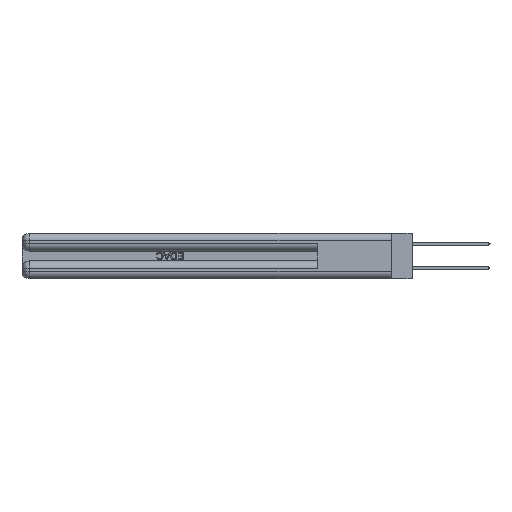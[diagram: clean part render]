
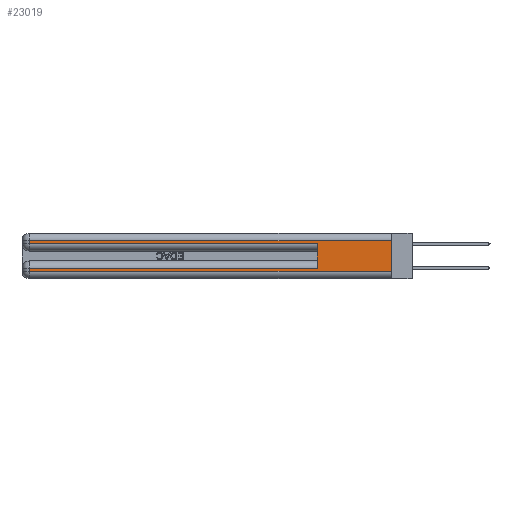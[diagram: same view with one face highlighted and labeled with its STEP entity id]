
A CAD part, left-side view. The second image highlights one B-rep face of the part: STEP entity #23019.
In plain terms, the highlighted planar face has unit normal (-1, 0, 0).
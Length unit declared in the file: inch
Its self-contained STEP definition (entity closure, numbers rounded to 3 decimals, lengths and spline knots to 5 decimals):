
#2296 = VERTEX_POINT ( 'NONE', #18502 ) ;
#3712 = VECTOR ( 'NONE', #10971, 39.37008 ) ;
#4779 = DIRECTION ( 'NONE',  ( 0., 0., -1. ) ) ;
#4962 = LINE ( 'NONE', #7095, #3712 ) ;
#5182 = CARTESIAN_POINT ( 'NONE',  ( 0., 2.94, 0.37 ) ) ;
#5480 = EDGE_CURVE ( 'NONE', #11653, #17614, #48073, .T. ) ;
#6185 = ORIENTED_EDGE ( 'NONE', *, *, #13485, .F. ) ;
#7095 = CARTESIAN_POINT ( 'NONE',  ( 0., 0., 0.06 ) ) ;
#7738 = CARTESIAN_POINT ( 'NONE',  ( 0., 0.6, 0.285 ) ) ;
#10971 = DIRECTION ( 'NONE',  ( 0., -1., 0. ) ) ;
#11653 = VERTEX_POINT ( 'NONE', #35361 ) ;
#11912 = DIRECTION ( 'NONE',  ( 0., 1., 0. ) ) ;
#13485 = EDGE_CURVE ( 'NONE', #11653, #46406, #41781, .T. ) ;
#13730 = EDGE_CURVE ( 'NONE', #17614, #25439, #42348, .T. ) ;
#14300 = CARTESIAN_POINT ( 'NONE',  ( 0., 0., 0.37 ) ) ;
#14472 = ORIENTED_EDGE ( 'NONE', *, *, #40665, .T. ) ;
#14673 = EDGE_CURVE ( 'NONE', #25762, #19172, #30805, .T. ) ;
#16099 = LINE ( 'NONE', #44958, #44363 ) ;
#17614 = VERTEX_POINT ( 'NONE', #29592 ) ;
#18148 = DIRECTION ( 'NONE',  ( 0., 0., -1. ) ) ;
#18502 = CARTESIAN_POINT ( 'NONE',  ( 0., 2.94, 0.06 ) ) ;
#18577 = CARTESIAN_POINT ( 'NONE',  ( 0., 2.94, 0.37 ) ) ;
#19172 = VERTEX_POINT ( 'NONE', #7738 ) ;
#19810 = EDGE_CURVE ( 'NONE', #2296, #46406, #4962, .T. ) ;
#20044 = LINE ( 'NONE', #18577, #49544 ) ;
#20166 = LINE ( 'NONE', #48658, #39418 ) ;
#20925 = ORIENTED_EDGE ( 'NONE', *, *, #19810, .T. ) ;
#21253 = DIRECTION ( 'NONE',  ( 0., 0., 1. ) ) ;
#22101 = ORIENTED_EDGE ( 'NONE', *, *, #5480, .T. ) ;
#22471 = DIRECTION ( 'NONE',  ( 0., 0., -1. ) ) ;
#23019 = ADVANCED_FACE ( 'NONE', ( #25878 ), #37299, .F. ) ;
#23479 = EDGE_LOOP ( 'NONE', ( #6185, #22101, #35210, #14472, #24970, #36206, #28091, #20925 ) ) ;
#24023 = VERTEX_POINT ( 'NONE', #25479 ) ;
#24338 = VECTOR ( 'NONE', #4779, 39.37008 ) ;
#24970 = ORIENTED_EDGE ( 'NONE', *, *, #14673, .F. ) ;
#25439 = VERTEX_POINT ( 'NONE', #44854 ) ;
#25479 = CARTESIAN_POINT ( 'NONE',  ( 0., 2.94, 0.085 ) ) ;
#25762 = VERTEX_POINT ( 'NONE', #31152 ) ;
#25878 = FACE_OUTER_BOUND ( 'NONE', #23479, .T. ) ;
#26979 = DIRECTION ( 'NONE',  ( 0., 0., -1. ) ) ;
#27255 = AXIS2_PLACEMENT_3D ( 'NONE', #14300, #41197, #18148 ) ;
#28091 = ORIENTED_EDGE ( 'NONE', *, *, #32267, .T. ) ;
#29592 = CARTESIAN_POINT ( 'NONE',  ( 0., 2.94, 0.31 ) ) ;
#29630 = DIRECTION ( 'NONE',  ( 0., 1., 0. ) ) ;
#29895 = EDGE_CURVE ( 'NONE', #25762, #24023, #16099, .T. ) ;
#30805 = LINE ( 'NONE', #48164, #39850 ) ;
#31152 = CARTESIAN_POINT ( 'NONE',  ( 0., 0.6, 0.085 ) ) ;
#32267 = EDGE_CURVE ( 'NONE', #24023, #2296, #20044, .T. ) ;
#32754 = VECTOR ( 'NONE', #26979, 39.37008 ) ;
#33334 = DIRECTION ( 'NONE',  ( 0., -1., 0. ) ) ;
#34936 = CARTESIAN_POINT ( 'NONE',  ( 0., 0., 0.31 ) ) ;
#35210 = ORIENTED_EDGE ( 'NONE', *, *, #13730, .T. ) ;
#35361 = CARTESIAN_POINT ( 'NONE',  ( 0., 0., 0.31 ) ) ;
#36206 = ORIENTED_EDGE ( 'NONE', *, *, #29895, .T. ) ;
#37299 = PLANE ( 'NONE',  #27255 ) ;
#39418 = VECTOR ( 'NONE', #33334, 39.37008 ) ;
#39850 = VECTOR ( 'NONE', #21253, 39.37008 ) ;
#40665 = EDGE_CURVE ( 'NONE', #25439, #19172, #20166, .T. ) ;
#41197 = DIRECTION ( 'NONE',  ( 1., 0., 0. ) ) ;
#41781 = LINE ( 'NONE', #46141, #32754 ) ;
#42348 = LINE ( 'NONE', #5182, #24338 ) ;
#43570 = CARTESIAN_POINT ( 'NONE',  ( 0., 0., 0.06 ) ) ;
#44363 = VECTOR ( 'NONE', #29630, 39.37008 ) ;
#44854 = CARTESIAN_POINT ( 'NONE',  ( 0., 2.94, 0.285 ) ) ;
#44958 = CARTESIAN_POINT ( 'NONE',  ( 0., 0., 0.085 ) ) ;
#46141 = CARTESIAN_POINT ( 'NONE',  ( 0., 0., 0.37 ) ) ;
#46406 = VERTEX_POINT ( 'NONE', #43570 ) ;
#46876 = VECTOR ( 'NONE', #11912, 39.37008 ) ;
#48073 = LINE ( 'NONE', #34936, #46876 ) ;
#48164 = CARTESIAN_POINT ( 'NONE',  ( 0., 0.6, 0.145 ) ) ;
#48658 = CARTESIAN_POINT ( 'NONE',  ( 0., 0., 0.285 ) ) ;
#49544 = VECTOR ( 'NONE', #22471, 39.37008 ) ;
